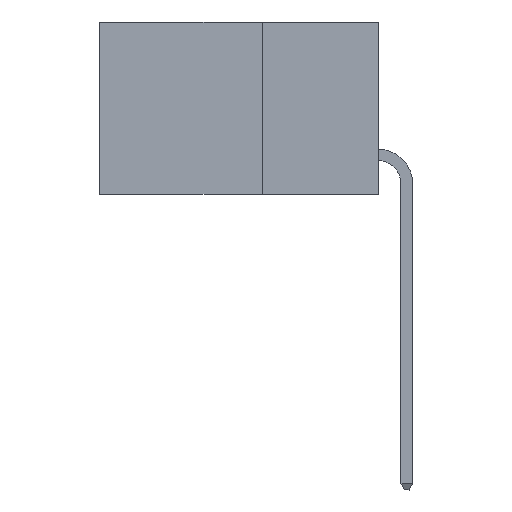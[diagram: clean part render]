
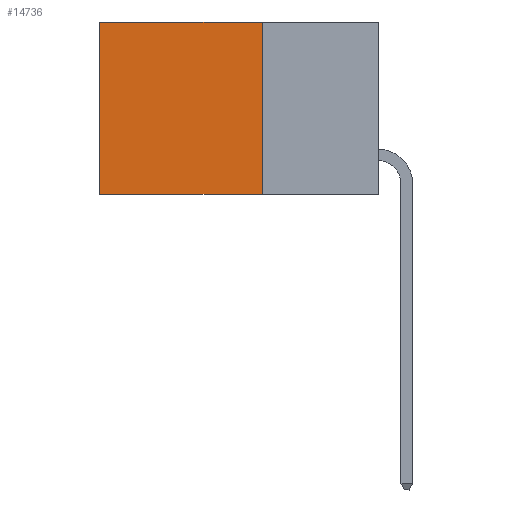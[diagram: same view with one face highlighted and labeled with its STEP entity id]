
A CAD part, left-side view. The second image highlights one B-rep face of the part: STEP entity #14736.
In plain terms, the highlighted planar face has unit normal (-1, 0, 0).
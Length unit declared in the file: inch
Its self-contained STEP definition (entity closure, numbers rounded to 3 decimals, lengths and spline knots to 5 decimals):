
#365 = VERTEX_POINT ( 'NONE', #7942 ) ;
#564 = PLANE ( 'NONE',  #18148 ) ;
#689 = ORIENTED_EDGE ( 'NONE', *, *, #23121, .T. ) ;
#1303 = EDGE_CURVE ( 'NONE', #16698, #18617, #14890, .T. ) ;
#2028 = DIRECTION ( 'NONE',  ( 0., 0., -1. ) ) ;
#2697 = CARTESIAN_POINT ( 'NONE',  ( 0.298, 0.25, 0. ) ) ;
#4857 = DIRECTION ( 'NONE',  ( 1., 0., 0. ) ) ;
#5032 = VECTOR ( 'NONE', #25715, 39.37008 ) ;
#5154 = ORIENTED_EDGE ( 'NONE', *, *, #9627, .F. ) ;
#5168 = ORIENTED_EDGE ( 'NONE', *, *, #1303, .T. ) ;
#5844 = LINE ( 'NONE', #12727, #11253 ) ;
#6673 = CARTESIAN_POINT ( 'NONE',  ( 0.298, 0.25, 0. ) ) ;
#6765 = DIRECTION ( 'NONE',  ( 0., 1., 0. ) ) ;
#7322 = EDGE_LOOP ( 'NONE', ( #5168, #5154, #23997, #689 ) ) ;
#7942 = CARTESIAN_POINT ( 'NONE',  ( 0.298, 0.25, 0. ) ) ;
#8433 = CARTESIAN_POINT ( 'NONE',  ( 0.298, 0.25, -0.37 ) ) ;
#8615 = CARTESIAN_POINT ( 'NONE',  ( 0.298, 0.6, -0.37 ) ) ;
#8623 = DIRECTION ( 'NONE',  ( 0., 0., -1. ) ) ;
#9627 = EDGE_CURVE ( 'NONE', #14004, #18617, #21790, .T. ) ;
#11253 = VECTOR ( 'NONE', #8623, 39.37008 ) ;
#12176 = CARTESIAN_POINT ( 'NONE',  ( 0.298, 0.6, 0. ) ) ;
#12538 = EDGE_CURVE ( 'NONE', #365, #14004, #5844, .T. ) ;
#12727 = CARTESIAN_POINT ( 'NONE',  ( 0.298, 0.25, 0. ) ) ;
#13064 = FACE_OUTER_BOUND ( 'NONE', #7322, .T. ) ;
#14004 = VERTEX_POINT ( 'NONE', #8433 ) ;
#14235 = VECTOR ( 'NONE', #2028, 39.37008 ) ;
#14736 = ADVANCED_FACE ( 'NONE', ( #13064 ), #564, .F. ) ;
#14890 = LINE ( 'NONE', #24724, #14235 ) ;
#16698 = VERTEX_POINT ( 'NONE', #12176 ) ;
#18148 = AXIS2_PLACEMENT_3D ( 'NONE', #2697, #4857, #18989 ) ;
#18617 = VERTEX_POINT ( 'NONE', #8615 ) ;
#18989 = DIRECTION ( 'NONE',  ( 0., 0., -1. ) ) ;
#21663 = CARTESIAN_POINT ( 'NONE',  ( 0.298, 0.25, -0.37 ) ) ;
#21790 = LINE ( 'NONE', #21663, #5032 ) ;
#23121 = EDGE_CURVE ( 'NONE', #365, #16698, #25502, .T. ) ;
#23997 = ORIENTED_EDGE ( 'NONE', *, *, #12538, .F. ) ;
#24724 = CARTESIAN_POINT ( 'NONE',  ( 0.298, 0.6, 0. ) ) ;
#24868 = VECTOR ( 'NONE', #6765, 39.37008 ) ;
#25502 = LINE ( 'NONE', #6673, #24868 ) ;
#25715 = DIRECTION ( 'NONE',  ( 0., 1., 0. ) ) ;
